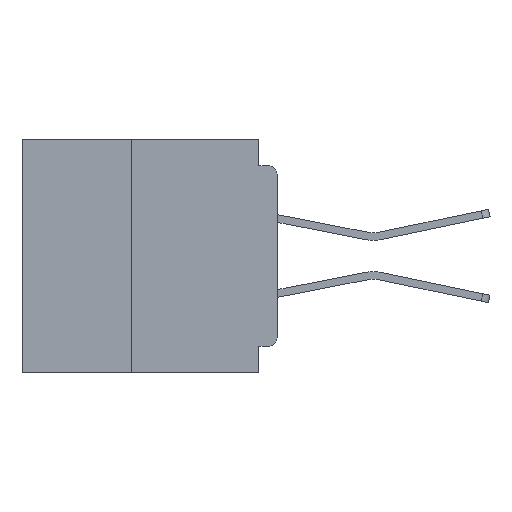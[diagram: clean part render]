
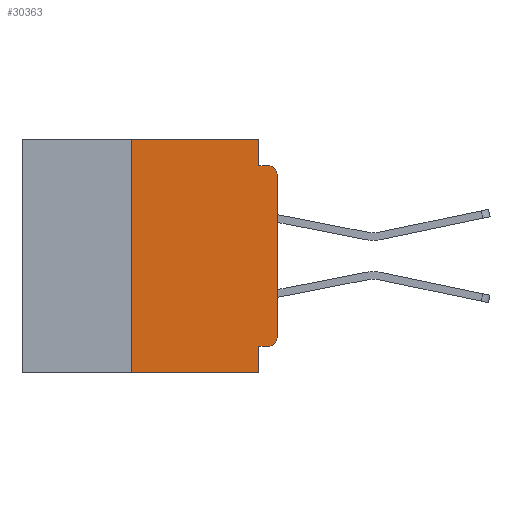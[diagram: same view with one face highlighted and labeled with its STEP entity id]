
A CAD part, left-side view. The second image highlights one B-rep face of the part: STEP entity #30363.
In plain terms, the highlighted planar face has unit normal (-1, 0, 0).
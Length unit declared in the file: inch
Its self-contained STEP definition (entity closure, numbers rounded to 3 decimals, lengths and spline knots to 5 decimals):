
#514 = ORIENTED_EDGE ( 'NONE', *, *, #30439, .F. ) ;
#1085 = EDGE_CURVE ( 'NONE', #1503, #35798, #36858, .T. ) ;
#1496 = CARTESIAN_POINT ( 'NONE',  ( 0., 0.031, -0.4 ) ) ;
#1503 = VERTEX_POINT ( 'NONE', #27963 ) ;
#2123 = CARTESIAN_POINT ( 'NONE',  ( 0., 0.031, 0. ) ) ;
#4023 = EDGE_CURVE ( 'NONE', #21280, #23592, #11246, .T. ) ;
#4310 = ORIENTED_EDGE ( 'NONE', *, *, #32122, .T. ) ;
#4424 = VECTOR ( 'NONE', #26162, 39.37008 ) ;
#4609 = DIRECTION ( 'NONE',  ( 0., 0., -1. ) ) ;
#5225 = ORIENTED_EDGE ( 'NONE', *, *, #22245, .T. ) ;
#5962 = CARTESIAN_POINT ( 'NONE',  ( 0., 0.031, 0. ) ) ;
#6878 = VECTOR ( 'NONE', #4609, 39.37008 ) ;
#6983 = DIRECTION ( 'NONE',  ( -1., 0., 0. ) ) ;
#8131 = CARTESIAN_POINT ( 'NONE',  ( 0., 0.031, -0.045 ) ) ;
#8768 = ORIENTED_EDGE ( 'NONE', *, *, #20669, .F. ) ;
#9077 = LINE ( 'NONE', #38931, #17194 ) ;
#9709 = CARTESIAN_POINT ( 'NONE',  ( 0., 0.437, -0.4 ) ) ;
#9982 = AXIS2_PLACEMENT_3D ( 'NONE', #28463, #16420, #37623 ) ;
#11246 = LINE ( 'NONE', #5962, #26438 ) ;
#12049 = CARTESIAN_POINT ( 'NONE',  ( 0., 0.015, -0.34 ) ) ;
#12152 = VERTEX_POINT ( 'NONE', #16100 ) ;
#12319 = VECTOR ( 'NONE', #33956, 39.37008 ) ;
#12469 = DIRECTION ( 'NONE',  ( 0., 0., 1. ) ) ;
#12485 = ORIENTED_EDGE ( 'NONE', *, *, #18695, .F. ) ;
#12776 = LINE ( 'NONE', #36728, #29837 ) ;
#13298 = LINE ( 'NONE', #33829, #12319 ) ;
#13934 = VERTEX_POINT ( 'NONE', #24328 ) ;
#14010 = CARTESIAN_POINT ( 'NONE',  ( 0., 0.25, -0.4 ) ) ;
#14312 = ORIENTED_EDGE ( 'NONE', *, *, #38765, .F. ) ;
#14594 = ORIENTED_EDGE ( 'NONE', *, *, #4023, .F. ) ;
#14694 = DIRECTION ( 'NONE',  ( 0., -1., 0. ) ) ;
#14805 = VERTEX_POINT ( 'NONE', #23388 ) ;
#15140 = DIRECTION ( 'NONE',  ( 0., 0., -1. ) ) ;
#15685 = ORIENTED_EDGE ( 'NONE', *, *, #22661, .F. ) ;
#16100 = CARTESIAN_POINT ( 'NONE',  ( 0., 0.25, 0. ) ) ;
#16420 = DIRECTION ( 'NONE',  ( 1., 0., 0. ) ) ;
#16522 = CARTESIAN_POINT ( 'NONE',  ( 0., 0.015, -0.355 ) ) ;
#17194 = VECTOR ( 'NONE', #14694, 39.37008 ) ;
#17973 = CIRCLE ( 'NONE', #22819, 0.015 ) ;
#18563 = VERTEX_POINT ( 'NONE', #16522 ) ;
#18695 = EDGE_CURVE ( 'NONE', #18563, #13934, #20677, .T. ) ;
#19503 = DIRECTION ( 'NONE',  ( 0., 0., -1. ) ) ;
#20436 = VECTOR ( 'NONE', #37079, 39.37008 ) ;
#20669 = EDGE_CURVE ( 'NONE', #23592, #34964, #9077, .T. ) ;
#20677 = LINE ( 'NONE', #32124, #4424 ) ;
#20726 = VECTOR ( 'NONE', #22374, 39.37008 ) ;
#21280 = VERTEX_POINT ( 'NONE', #2123 ) ;
#22245 = EDGE_CURVE ( 'NONE', #31230, #14805, #28488, .T. ) ;
#22374 = DIRECTION ( 'NONE',  ( 0., 0., 1. ) ) ;
#22661 = EDGE_CURVE ( 'NONE', #12152, #21280, #13298, .T. ) ;
#22819 = AXIS2_PLACEMENT_3D ( 'NONE', #25214, #6983, #28262 ) ;
#23388 = CARTESIAN_POINT ( 'NONE',  ( 0., 0.031, -0.4 ) ) ;
#23592 = VERTEX_POINT ( 'NONE', #8131 ) ;
#24328 = CARTESIAN_POINT ( 'NONE',  ( 0., 0.031, -0.355 ) ) ;
#25214 = CARTESIAN_POINT ( 'NONE',  ( 0., 0.015, -0.06 ) ) ;
#26162 = DIRECTION ( 'NONE',  ( 0., 1., 0. ) ) ;
#26438 = VECTOR ( 'NONE', #19503, 39.37008 ) ;
#26493 = ORIENTED_EDGE ( 'NONE', *, *, #1085, .T. ) ;
#26748 = CIRCLE ( 'NONE', #38797, 0.015 ) ;
#27963 = CARTESIAN_POINT ( 'NONE',  ( 0., 0., -0.34 ) ) ;
#28262 = DIRECTION ( 'NONE',  ( 0., 0., -1. ) ) ;
#28463 = CARTESIAN_POINT ( 'NONE',  ( 0., 0.437, 0. ) ) ;
#28488 = LINE ( 'NONE', #9709, #20436 ) ;
#29378 = EDGE_LOOP ( 'NONE', ( #26493, #33785, #8768, #14594, #15685, #14312, #5225, #514, #12485, #4310 ) ) ;
#29837 = VECTOR ( 'NONE', #12469, 39.37008 ) ;
#30363 = ADVANCED_FACE ( 'NONE', ( #34962 ), #31500, .F. ) ;
#30436 = CARTESIAN_POINT ( 'NONE',  ( 0., 0.015, -0.045 ) ) ;
#30439 = EDGE_CURVE ( 'NONE', #13934, #14805, #31129, .T. ) ;
#31129 = LINE ( 'NONE', #1496, #6878 ) ;
#31230 = VERTEX_POINT ( 'NONE', #14010 ) ;
#31500 = PLANE ( 'NONE',  #9982 ) ;
#32122 = EDGE_CURVE ( 'NONE', #18563, #1503, #26748, .T. ) ;
#32124 = CARTESIAN_POINT ( 'NONE',  ( 0., 0., -0.355 ) ) ;
#33257 = DIRECTION ( 'NONE',  ( -1., 0., 0. ) ) ;
#33519 = EDGE_CURVE ( 'NONE', #35798, #34964, #17973, .T. ) ;
#33785 = ORIENTED_EDGE ( 'NONE', *, *, #33519, .T. ) ;
#33829 = CARTESIAN_POINT ( 'NONE',  ( 0., 0.437, 0. ) ) ;
#33956 = DIRECTION ( 'NONE',  ( 0., -1., 0. ) ) ;
#34917 = CARTESIAN_POINT ( 'NONE',  ( 0., 0., -0.06 ) ) ;
#34962 = FACE_OUTER_BOUND ( 'NONE', #29378, .T. ) ;
#34964 = VERTEX_POINT ( 'NONE', #30436 ) ;
#35798 = VERTEX_POINT ( 'NONE', #34917 ) ;
#36728 = CARTESIAN_POINT ( 'NONE',  ( 0., 0.25, -0.4 ) ) ;
#36858 = LINE ( 'NONE', #39347, #20726 ) ;
#37079 = DIRECTION ( 'NONE',  ( 0., -1., 0. ) ) ;
#37623 = DIRECTION ( 'NONE',  ( 0., 0., -1. ) ) ;
#38765 = EDGE_CURVE ( 'NONE', #31230, #12152, #12776, .T. ) ;
#38797 = AXIS2_PLACEMENT_3D ( 'NONE', #12049, #33257, #15140 ) ;
#38931 = CARTESIAN_POINT ( 'NONE',  ( 0., 0., -0.045 ) ) ;
#39347 = CARTESIAN_POINT ( 'NONE',  ( 0., 0., 0. ) ) ;
